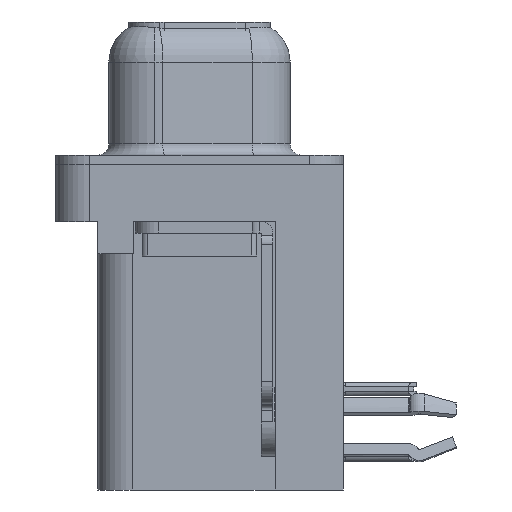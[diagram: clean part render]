
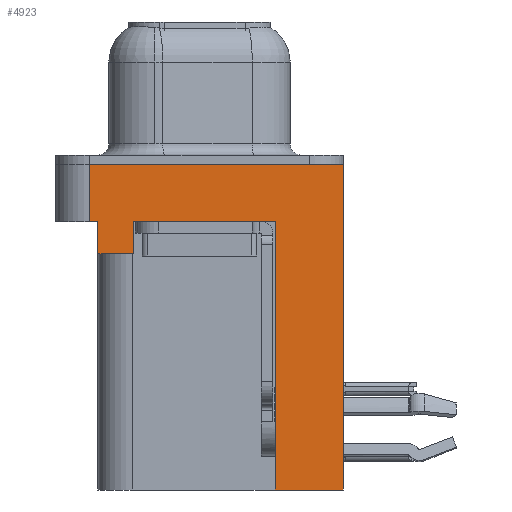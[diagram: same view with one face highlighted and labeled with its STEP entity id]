
A CAD part, left-side view. The second image highlights one B-rep face of the part: STEP entity #4923.
In plain terms, the highlighted planar face has unit normal (-1, 0, 0).
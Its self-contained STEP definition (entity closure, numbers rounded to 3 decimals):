
#341 = VERTEX_POINT ( 'NONE', #9596 ) ;
#603 = ORIENTED_EDGE ( 'NONE', *, *, #21020, .F. ) ;
#758 = EDGE_CURVE ( 'NONE', #6771, #1855, #22736, .T. ) ;
#763 = VECTOR ( 'NONE', #9607, 1000. ) ;
#1041 = CARTESIAN_POINT ( 'NONE',  ( -2.935, 4.775, -2.5 ) ) ;
#1149 = VERTEX_POINT ( 'NONE', #1041 ) ;
#1222 = CARTESIAN_POINT ( 'NONE',  ( -2.935, -6.275, -2.5 ) ) ;
#1571 = LINE ( 'NONE', #9702, #24929 ) ;
#1580 = EDGE_CURVE ( 'NONE', #16707, #341, #7549, .T. ) ;
#1612 = CARTESIAN_POINT ( 'NONE',  ( -2.935, 4.425, -3.9 ) ) ;
#1705 = DIRECTION ( 'NONE',  ( 0., -1., 0. ) ) ;
#1766 = DIRECTION ( 'NONE',  ( 0., -1., 0. ) ) ;
#1855 = VERTEX_POINT ( 'NONE', #18580 ) ;
#1968 = LINE ( 'NONE', #8399, #2737 ) ;
#2049 = CARTESIAN_POINT ( 'NONE',  ( -2.935, 2.895, -3.9 ) ) ;
#2687 = VECTOR ( 'NONE', #25491, 1000. ) ;
#2737 = VECTOR ( 'NONE', #10103, 1000. ) ;
#3455 = LINE ( 'NONE', #1612, #763 ) ;
#4502 = LINE ( 'NONE', #16087, #6668 ) ;
#4780 = LINE ( 'NONE', #19459, #2687 ) ;
#4875 = ORIENTED_EDGE ( 'NONE', *, *, #22544, .F. ) ;
#4923 = ADVANCED_FACE ( 'NONE', ( #13039 ), #15275, .T. ) ;
#5128 = DIRECTION ( 'NONE',  ( 0., 0., 1. ) ) ;
#5131 = CARTESIAN_POINT ( 'NONE',  ( -2.935, -6.275, 0. ) ) ;
#5380 = DIRECTION ( 'NONE',  ( 0., 0., 1. ) ) ;
#5864 = LINE ( 'NONE', #2049, #7899 ) ;
#5915 = VERTEX_POINT ( 'NONE', #12693 ) ;
#6147 = CARTESIAN_POINT ( 'NONE',  ( -2.935, 4.775, 0. ) ) ;
#6668 = VECTOR ( 'NONE', #18579, 1000. ) ;
#6741 = VERTEX_POINT ( 'NONE', #7976 ) ;
#6771 = VERTEX_POINT ( 'NONE', #21656 ) ;
#7544 = CARTESIAN_POINT ( 'NONE',  ( -2.935, 2.895, -2.5 ) ) ;
#7549 = LINE ( 'NONE', #19776, #12288 ) ;
#7589 = ORIENTED_EDGE ( 'NONE', *, *, #12859, .T. ) ;
#7899 = VECTOR ( 'NONE', #14139, 1000. ) ;
#7949 = EDGE_CURVE ( 'NONE', #21471, #5915, #15108, .T. ) ;
#7976 = CARTESIAN_POINT ( 'NONE',  ( -2.935, 2.895, -3.9 ) ) ;
#8036 = EDGE_CURVE ( 'NONE', #17390, #341, #1571, .T. ) ;
#8227 = ORIENTED_EDGE ( 'NONE', *, *, #758, .F. ) ;
#8399 = CARTESIAN_POINT ( 'NONE',  ( -2.935, 4.775, -2.5 ) ) ;
#9354 = DIRECTION ( 'NONE',  ( 0., 0., 1. ) ) ;
#9596 = CARTESIAN_POINT ( 'NONE',  ( -2.935, -3.295, -2.5 ) ) ;
#9607 = DIRECTION ( 'NONE',  ( 0., 1., 0. ) ) ;
#9702 = CARTESIAN_POINT ( 'NONE',  ( -2.935, -3.295, -14.2 ) ) ;
#9784 = ORIENTED_EDGE ( 'NONE', *, *, #7949, .T. ) ;
#9844 = VECTOR ( 'NONE', #5128, 1000. ) ;
#10103 = DIRECTION ( 'NONE',  ( 0., 0., 1. ) ) ;
#10162 = EDGE_CURVE ( 'NONE', #6741, #6771, #3455, .T. ) ;
#11297 = VECTOR ( 'NONE', #24711, 1000. ) ;
#11360 = ORIENTED_EDGE ( 'NONE', *, *, #1580, .T. ) ;
#12288 = VECTOR ( 'NONE', #1766, 1000. ) ;
#12693 = CARTESIAN_POINT ( 'NONE',  ( -2.935, -6.275, 0. ) ) ;
#12859 = EDGE_CURVE ( 'NONE', #6741, #16707, #5864, .T. ) ;
#12947 = AXIS2_PLACEMENT_3D ( 'NONE', #1222, #25523, #9354 ) ;
#13039 = FACE_OUTER_BOUND ( 'NONE', #15892, .T. ) ;
#13152 = EDGE_CURVE ( 'NONE', #21471, #17390, #4502, .T. ) ;
#14139 = DIRECTION ( 'NONE',  ( 0., 0., 1. ) ) ;
#14799 = ORIENTED_EDGE ( 'NONE', *, *, #13152, .F. ) ;
#15108 = LINE ( 'NONE', #16961, #9844 ) ;
#15275 = PLANE ( 'NONE',  #12947 ) ;
#15892 = EDGE_LOOP ( 'NONE', ( #603, #4875, #24791, #8227, #19943, #7589, #11360, #19742, #14799, #9784 ) ) ;
#16087 = CARTESIAN_POINT ( 'NONE',  ( -2.935, -3.295, -14.2 ) ) ;
#16549 = CARTESIAN_POINT ( 'NONE',  ( -2.935, -6.275, -14.2 ) ) ;
#16707 = VERTEX_POINT ( 'NONE', #7544 ) ;
#16961 = CARTESIAN_POINT ( 'NONE',  ( -2.935, -6.275, -2.5 ) ) ;
#17078 = CARTESIAN_POINT ( 'NONE',  ( -2.935, 4.425, -3.9 ) ) ;
#17390 = VERTEX_POINT ( 'NONE', #21752 ) ;
#18579 = DIRECTION ( 'NONE',  ( 0., 1., 0. ) ) ;
#18580 = CARTESIAN_POINT ( 'NONE',  ( -2.935, 4.425, -2.5 ) ) ;
#19459 = CARTESIAN_POINT ( 'NONE',  ( -2.935, -6.275, -2.5 ) ) ;
#19579 = LINE ( 'NONE', #5131, #21969 ) ;
#19742 = ORIENTED_EDGE ( 'NONE', *, *, #8036, .F. ) ;
#19776 = CARTESIAN_POINT ( 'NONE',  ( -2.935, -6.275, -2.5 ) ) ;
#19943 = ORIENTED_EDGE ( 'NONE', *, *, #10162, .F. ) ;
#20971 = EDGE_CURVE ( 'NONE', #1149, #1855, #4780, .T. ) ;
#21020 = EDGE_CURVE ( 'NONE', #23106, #5915, #19579, .T. ) ;
#21471 = VERTEX_POINT ( 'NONE', #16549 ) ;
#21656 = CARTESIAN_POINT ( 'NONE',  ( -2.935, 4.425, -3.9 ) ) ;
#21752 = CARTESIAN_POINT ( 'NONE',  ( -2.935, -3.295, -14.2 ) ) ;
#21969 = VECTOR ( 'NONE', #1705, 1000. ) ;
#22544 = EDGE_CURVE ( 'NONE', #1149, #23106, #1968, .T. ) ;
#22736 = LINE ( 'NONE', #17078, #11297 ) ;
#23106 = VERTEX_POINT ( 'NONE', #6147 ) ;
#24711 = DIRECTION ( 'NONE',  ( 0., 0., 1. ) ) ;
#24791 = ORIENTED_EDGE ( 'NONE', *, *, #20971, .T. ) ;
#24929 = VECTOR ( 'NONE', #5380, 1000. ) ;
#25491 = DIRECTION ( 'NONE',  ( 0., -1., 0. ) ) ;
#25523 = DIRECTION ( 'NONE',  ( -1., 0., 0. ) ) ;
